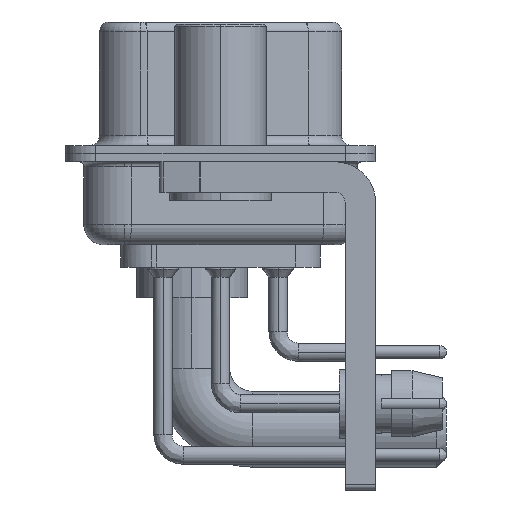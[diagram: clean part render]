
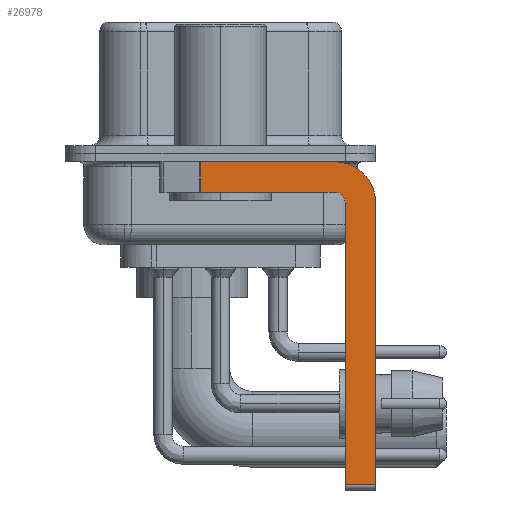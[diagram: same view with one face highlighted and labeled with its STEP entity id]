
A CAD part, left-side view. The second image highlights one B-rep face of the part: STEP entity #26978.
In plain terms, the highlighted planar face has unit normal (-1, 0, 0).
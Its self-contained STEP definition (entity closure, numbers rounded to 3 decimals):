
#1347 = CARTESIAN_POINT ( 'NONE',  ( -2.9, -5.65, -2.4 ) ) ;
#1552 = ORIENTED_EDGE ( 'NONE', *, *, #29879, .F. ) ;
#1553 = DIRECTION ( 'NONE',  ( 0., 0., -1. ) ) ;
#1761 = VECTOR ( 'NONE', #10798, 1000. ) ;
#2619 = ORIENTED_EDGE ( 'NONE', *, *, #33821, .F. ) ;
#4705 = CARTESIAN_POINT ( 'NONE',  ( -2.9, 0.978, -1.9 ) ) ;
#5422 = DIRECTION ( 'NONE',  ( 0., 0., -1. ) ) ;
#5749 = VERTEX_POINT ( 'NONE', #32049 ) ;
#6433 = EDGE_CURVE ( 'NONE', #16603, #20439, #32489, .T. ) ;
#6974 = LINE ( 'NONE', #35556, #8317 ) ;
#7220 = VECTOR ( 'NONE', #27188, 1000. ) ;
#7573 = AXIS2_PLACEMENT_3D ( 'NONE', #1347, #14168, #1553 ) ;
#8178 = CARTESIAN_POINT ( 'NONE',  ( -2.9, -5.65, -16.35 ) ) ;
#8317 = VECTOR ( 'NONE', #32612, 1000. ) ;
#8806 = LINE ( 'NONE', #8178, #27034 ) ;
#9040 = CARTESIAN_POINT ( 'NONE',  ( -2.9, -5.65, -0.4 ) ) ;
#10146 = CARTESIAN_POINT ( 'NONE',  ( -2.9, 0.978, -0.4 ) ) ;
#10288 = CARTESIAN_POINT ( 'NONE',  ( -2.9, -5.65, -2.4 ) ) ;
#10704 = EDGE_CURVE ( 'NONE', #39666, #37962, #6974, .T. ) ;
#10798 = DIRECTION ( 'NONE',  ( 0., 0., 1. ) ) ;
#11576 = AXIS2_PLACEMENT_3D ( 'NONE', #10288, #33191, #13852 ) ;
#11803 = CARTESIAN_POINT ( 'NONE',  ( -2.9, -6.15, -2.4 ) ) ;
#13152 = CARTESIAN_POINT ( 'NONE',  ( -2.9, -5.65, -1.9 ) ) ;
#13852 = DIRECTION ( 'NONE',  ( 0., 0., -1. ) ) ;
#13874 = EDGE_CURVE ( 'NONE', #5749, #31801, #36840, .T. ) ;
#14168 = DIRECTION ( 'NONE',  ( 1., 0., 0. ) ) ;
#14844 = CARTESIAN_POINT ( 'NONE',  ( -2.9, 0.978, -1.9 ) ) ;
#15778 = CARTESIAN_POINT ( 'NONE',  ( -2.9, -7.65, -16.35 ) ) ;
#16603 = VERTEX_POINT ( 'NONE', #40138 ) ;
#16944 = DIRECTION ( 'NONE',  ( 0., 0., 1. ) ) ;
#17355 = CARTESIAN_POINT ( 'NONE',  ( -2.9, -5.65, -2.4 ) ) ;
#18732 = VERTEX_POINT ( 'NONE', #15778 ) ;
#20439 = VERTEX_POINT ( 'NONE', #14844 ) ;
#20841 = EDGE_CURVE ( 'NONE', #39666, #20439, #37066, .T. ) ;
#20858 = CARTESIAN_POINT ( 'NONE',  ( -2.9, -6.15, -16.6 ) ) ;
#23032 = EDGE_LOOP ( 'NONE', ( #39487, #35103, #30695, #2619, #35208, #30597, #1552, #36645 ) ) ;
#23459 = DIRECTION ( 'NONE',  ( -1., 0., 0. ) ) ;
#24542 = VECTOR ( 'NONE', #5422, 1000. ) ;
#26352 = VECTOR ( 'NONE', #38778, 1000. ) ;
#26978 = ADVANCED_FACE ( 'NONE', ( #36550 ), #39064, .F. ) ;
#27034 = VECTOR ( 'NONE', #30674, 1000. ) ;
#27161 = EDGE_CURVE ( 'NONE', #5749, #18732, #8806, .T. ) ;
#27188 = DIRECTION ( 'NONE',  ( 0., 0., -1. ) ) ;
#27487 = EDGE_CURVE ( 'NONE', #37962, #34553, #34430, .T. ) ;
#27935 = AXIS2_PLACEMENT_3D ( 'NONE', #17355, #23459, #16944 ) ;
#29879 = EDGE_CURVE ( 'NONE', #34553, #18732, #34417, .T. ) ;
#30597 = ORIENTED_EDGE ( 'NONE', *, *, #27161, .T. ) ;
#30674 = DIRECTION ( 'NONE',  ( 0., -1., 0. ) ) ;
#30695 = ORIENTED_EDGE ( 'NONE', *, *, #6433, .F. ) ;
#31801 = VERTEX_POINT ( 'NONE', #11803 ) ;
#31802 = CARTESIAN_POINT ( 'NONE',  ( -2.9, -7.65, -2.4 ) ) ;
#32049 = CARTESIAN_POINT ( 'NONE',  ( -2.9, -6.15, -16.35 ) ) ;
#32489 = LINE ( 'NONE', #13152, #26352 ) ;
#32612 = DIRECTION ( 'NONE',  ( 0., -1., 0. ) ) ;
#33191 = DIRECTION ( 'NONE',  ( 1., 0., 0. ) ) ;
#33821 = EDGE_CURVE ( 'NONE', #31801, #16603, #41331, .T. ) ;
#34417 = LINE ( 'NONE', #36937, #24542 ) ;
#34430 = CIRCLE ( 'NONE', #7573, 2. ) ;
#34553 = VERTEX_POINT ( 'NONE', #31802 ) ;
#35103 = ORIENTED_EDGE ( 'NONE', *, *, #20841, .T. ) ;
#35208 = ORIENTED_EDGE ( 'NONE', *, *, #13874, .F. ) ;
#35556 = CARTESIAN_POINT ( 'NONE',  ( -2.9, 3., -0.4 ) ) ;
#36550 = FACE_OUTER_BOUND ( 'NONE', #23032, .T. ) ;
#36645 = ORIENTED_EDGE ( 'NONE', *, *, #27487, .F. ) ;
#36840 = LINE ( 'NONE', #20858, #1761 ) ;
#36937 = CARTESIAN_POINT ( 'NONE',  ( -2.9, -7.65, -2.4 ) ) ;
#37066 = LINE ( 'NONE', #4705, #7220 ) ;
#37962 = VERTEX_POINT ( 'NONE', #9040 ) ;
#38778 = DIRECTION ( 'NONE',  ( 0., 1., 0. ) ) ;
#39064 = PLANE ( 'NONE',  #11576 ) ;
#39487 = ORIENTED_EDGE ( 'NONE', *, *, #10704, .F. ) ;
#39666 = VERTEX_POINT ( 'NONE', #10146 ) ;
#40138 = CARTESIAN_POINT ( 'NONE',  ( -2.9, -5.65, -1.9 ) ) ;
#41331 = CIRCLE ( 'NONE', #27935, 0.5 ) ;
